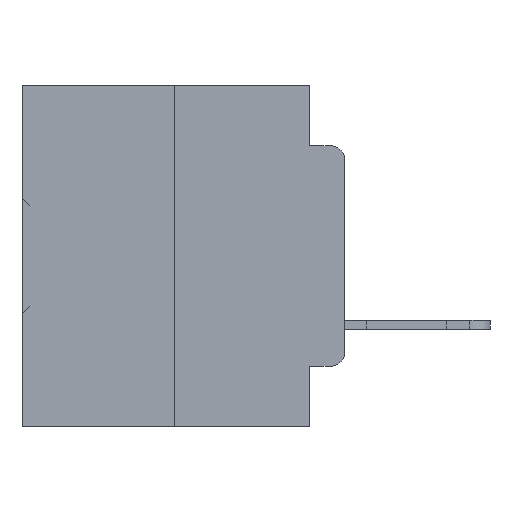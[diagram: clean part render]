
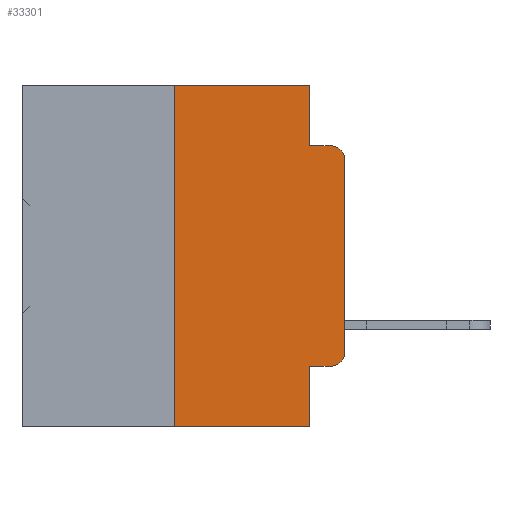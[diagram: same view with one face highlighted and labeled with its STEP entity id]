
A CAD part, left-side view. The second image highlights one B-rep face of the part: STEP entity #33301.
In plain terms, the highlighted planar face has unit normal (-1, 0, 0).
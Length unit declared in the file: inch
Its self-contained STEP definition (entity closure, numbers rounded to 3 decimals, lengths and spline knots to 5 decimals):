
#1785 = CARTESIAN_POINT ( 'NONE',  ( 0., 0.02, -0.4115 ) ) ;
#2602 = VERTEX_POINT ( 'NONE', #34862 ) ;
#3379 = CARTESIAN_POINT ( 'NONE',  ( 0., 0.02, -0.1085 ) ) ;
#3619 = LINE ( 'NONE', #22436, #33998 ) ;
#4254 = VERTEX_POINT ( 'NONE', #1785 ) ;
#4519 = VERTEX_POINT ( 'NONE', #11158 ) ;
#4898 = DIRECTION ( 'NONE',  ( 0., 0., 1. ) ) ;
#5297 = ORIENTED_EDGE ( 'NONE', *, *, #21869, .F. ) ;
#5878 = ORIENTED_EDGE ( 'NONE', *, *, #22203, .F. ) ;
#6045 = CARTESIAN_POINT ( 'NONE',  ( 0., 0.051, -0.5 ) ) ;
#6379 = DIRECTION ( 'NONE',  ( 0., 0., -1. ) ) ;
#7323 = CARTESIAN_POINT ( 'NONE',  ( 0., 0.02, -0.0885 ) ) ;
#7430 = CARTESIAN_POINT ( 'NONE',  ( 0., 0.473, 0. ) ) ;
#8536 = FACE_OUTER_BOUND ( 'NONE', #24137, .T. ) ;
#10680 = CARTESIAN_POINT ( 'NONE',  ( 0., 0.051, -0.0885 ) ) ;
#10691 = VERTEX_POINT ( 'NONE', #25025 ) ;
#10889 = DIRECTION ( 'NONE',  ( 0., -1., 0. ) ) ;
#11158 = CARTESIAN_POINT ( 'NONE',  ( 0., 0.25, 0. ) ) ;
#11300 = DIRECTION ( 'NONE',  ( 0., -1., 0. ) ) ;
#11399 = LINE ( 'NONE', #35694, #34645 ) ;
#11582 = VECTOR ( 'NONE', #21963, 39.37008 ) ;
#11894 = CIRCLE ( 'NONE', #30202, 0.02 ) ;
#13903 = CARTESIAN_POINT ( 'NONE',  ( 0., 0.051, -0.0885 ) ) ;
#14258 = CARTESIAN_POINT ( 'NONE',  ( 0., 0., -0.3915 ) ) ;
#14461 = ORIENTED_EDGE ( 'NONE', *, *, #24608, .T. ) ;
#15023 = VERTEX_POINT ( 'NONE', #36866 ) ;
#15129 = LINE ( 'NONE', #20220, #21969 ) ;
#16038 = EDGE_CURVE ( 'NONE', #15023, #24726, #23719, .T. ) ;
#16675 = CARTESIAN_POINT ( 'NONE',  ( 0., 0.02, -0.3915 ) ) ;
#17536 = LINE ( 'NONE', #21065, #24397 ) ;
#18410 = DIRECTION ( 'NONE',  ( 0., -1., 0. ) ) ;
#18621 = ORIENTED_EDGE ( 'NONE', *, *, #32896, .F. ) ;
#19184 = ORIENTED_EDGE ( 'NONE', *, *, #16038, .T. ) ;
#19193 = VECTOR ( 'NONE', #4898, 39.37008 ) ;
#19610 = DIRECTION ( 'NONE',  ( 0., 0., -1. ) ) ;
#19734 = AXIS2_PLACEMENT_3D ( 'NONE', #3379, #24051, #6379 ) ;
#20220 = CARTESIAN_POINT ( 'NONE',  ( 0., 0.051, -0.4115 ) ) ;
#21065 = CARTESIAN_POINT ( 'NONE',  ( 0., 0.051, 0. ) ) ;
#21189 = DIRECTION ( 'NONE',  ( 0., 0., -1. ) ) ;
#21869 = EDGE_CURVE ( 'NONE', #10691, #24726, #3619, .T. ) ;
#21873 = EDGE_CURVE ( 'NONE', #15023, #4519, #34829, .T. ) ;
#21934 = EDGE_CURVE ( 'NONE', #30446, #26149, #17536, .T. ) ;
#21963 = DIRECTION ( 'NONE',  ( 0., 0., 1. ) ) ;
#21969 = VECTOR ( 'NONE', #11300, 39.37008 ) ;
#22040 = CARTESIAN_POINT ( 'NONE',  ( 0., 0.25, 0. ) ) ;
#22120 = DIRECTION ( 'NONE',  ( 1., 0., 0. ) ) ;
#22131 = DIRECTION ( 'NONE',  ( 0., 0., -1. ) ) ;
#22203 = EDGE_CURVE ( 'NONE', #26149, #27557, #29031, .T. ) ;
#22252 = ORIENTED_EDGE ( 'NONE', *, *, #24436, .T. ) ;
#22436 = CARTESIAN_POINT ( 'NONE',  ( 0., 0.051, 0. ) ) ;
#23038 = VECTOR ( 'NONE', #10889, 39.37008 ) ;
#23719 = LINE ( 'NONE', #28473, #30616 ) ;
#24051 = DIRECTION ( 'NONE',  ( -1., 0., 0. ) ) ;
#24137 = EDGE_LOOP ( 'NONE', ( #29414, #34735, #5878, #36083, #18621, #32548, #19184, #5297, #14461, #22252 ) ) ;
#24397 = VECTOR ( 'NONE', #21189, 39.37008 ) ;
#24436 = EDGE_CURVE ( 'NONE', #4254, #31391, #11894, .T. ) ;
#24608 = EDGE_CURVE ( 'NONE', #10691, #4254, #15129, .T. ) ;
#24726 = VERTEX_POINT ( 'NONE', #6045 ) ;
#25025 = CARTESIAN_POINT ( 'NONE',  ( 0., 0.051, -0.4115 ) ) ;
#26054 = CIRCLE ( 'NONE', #19734, 0.02 ) ;
#26149 = VERTEX_POINT ( 'NONE', #13903 ) ;
#27015 = LINE ( 'NONE', #31339, #19193 ) ;
#27314 = AXIS2_PLACEMENT_3D ( 'NONE', #7430, #22120, #33857 ) ;
#27557 = VERTEX_POINT ( 'NONE', #7323 ) ;
#28146 = EDGE_CURVE ( 'NONE', #31391, #2602, #27015, .T. ) ;
#28473 = CARTESIAN_POINT ( 'NONE',  ( 0., 0.473, -0.5 ) ) ;
#28811 = DIRECTION ( 'NONE',  ( 0., -1., 0. ) ) ;
#29031 = LINE ( 'NONE', #10680, #23038 ) ;
#29061 = EDGE_CURVE ( 'NONE', #2602, #27557, #26054, .T. ) ;
#29414 = ORIENTED_EDGE ( 'NONE', *, *, #28146, .T. ) ;
#30202 = AXIS2_PLACEMENT_3D ( 'NONE', #16675, #36755, #19610 ) ;
#30446 = VERTEX_POINT ( 'NONE', #32651 ) ;
#30616 = VECTOR ( 'NONE', #28811, 39.37008 ) ;
#30990 = PLANE ( 'NONE',  #27314 ) ;
#31339 = CARTESIAN_POINT ( 'NONE',  ( 0., 0., 0. ) ) ;
#31391 = VERTEX_POINT ( 'NONE', #14258 ) ;
#32548 = ORIENTED_EDGE ( 'NONE', *, *, #21873, .F. ) ;
#32651 = CARTESIAN_POINT ( 'NONE',  ( 0., 0.051, 0. ) ) ;
#32896 = EDGE_CURVE ( 'NONE', #4519, #30446, #11399, .T. ) ;
#33301 = ADVANCED_FACE ( 'NONE', ( #8536 ), #30990, .F. ) ;
#33857 = DIRECTION ( 'NONE',  ( 0., 0., -1. ) ) ;
#33998 = VECTOR ( 'NONE', #22131, 39.37008 ) ;
#34645 = VECTOR ( 'NONE', #18410, 39.37008 ) ;
#34735 = ORIENTED_EDGE ( 'NONE', *, *, #29061, .T. ) ;
#34829 = LINE ( 'NONE', #22040, #11582 ) ;
#34862 = CARTESIAN_POINT ( 'NONE',  ( 0., 0., -0.1085 ) ) ;
#35694 = CARTESIAN_POINT ( 'NONE',  ( 0., 0.473, 0. ) ) ;
#36083 = ORIENTED_EDGE ( 'NONE', *, *, #21934, .F. ) ;
#36755 = DIRECTION ( 'NONE',  ( -1., 0., 0. ) ) ;
#36866 = CARTESIAN_POINT ( 'NONE',  ( 0., 0.25, -0.5 ) ) ;
